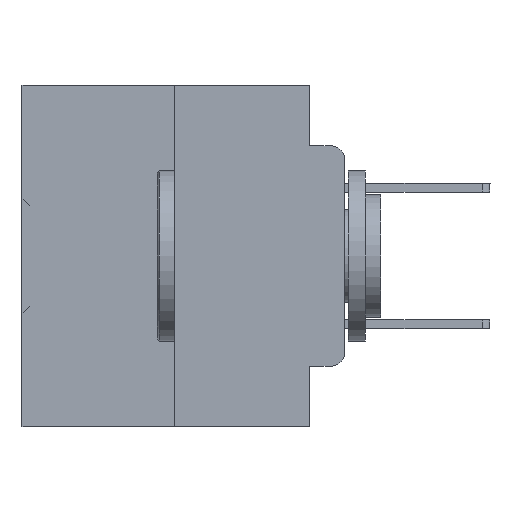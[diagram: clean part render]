
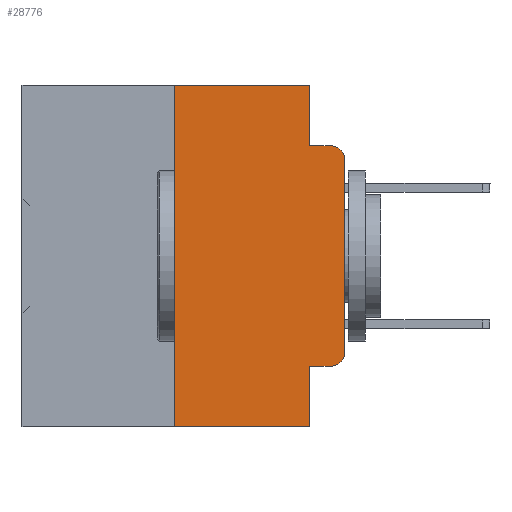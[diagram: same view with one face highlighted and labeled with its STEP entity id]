
A CAD part, left-side view. The second image highlights one B-rep face of the part: STEP entity #28776.
In plain terms, the highlighted planar face has unit normal (-1, 0, 0).
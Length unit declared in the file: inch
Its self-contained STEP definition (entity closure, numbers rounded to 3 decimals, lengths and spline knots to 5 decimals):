
#138 = VERTEX_POINT ( 'NONE', #4780 ) ;
#224 = VERTEX_POINT ( 'NONE', #30484 ) ;
#926 = VERTEX_POINT ( 'NONE', #33487 ) ;
#1005 = FACE_OUTER_BOUND ( 'NONE', #6523, .T. ) ;
#1361 = LINE ( 'NONE', #36546, #33646 ) ;
#1644 = CARTESIAN_POINT ( 'NONE',  ( 0., 0.02, -0.0885 ) ) ;
#2050 = CARTESIAN_POINT ( 'NONE',  ( 0., 0.02, -0.4115 ) ) ;
#2787 = DIRECTION ( 'NONE',  ( 0., 0., -1. ) ) ;
#3544 = EDGE_CURVE ( 'NONE', #7871, #9605, #33905, .T. ) ;
#3563 = ORIENTED_EDGE ( 'NONE', *, *, #5398, .F. ) ;
#4610 = CARTESIAN_POINT ( 'NONE',  ( 0., 0.051, -0.4115 ) ) ;
#4780 = CARTESIAN_POINT ( 'NONE',  ( 0., 0.051, 0. ) ) ;
#4832 = EDGE_CURVE ( 'NONE', #22934, #23309, #10709, .T. ) ;
#5270 = CARTESIAN_POINT ( 'NONE',  ( 0., 0.051, -0.0885 ) ) ;
#5398 = EDGE_CURVE ( 'NONE', #7871, #926, #38630, .T. ) ;
#5554 = CARTESIAN_POINT ( 'NONE',  ( 0., 0.02, -0.1085 ) ) ;
#5625 = LINE ( 'NONE', #5270, #18079 ) ;
#5853 = VECTOR ( 'NONE', #7792, 39.37008 ) ;
#6523 = EDGE_LOOP ( 'NONE', ( #37694, #24678, #22827, #24062, #15178, #3563, #34292, #28513, #22825, #31174 ) ) ;
#6553 = VECTOR ( 'NONE', #20130, 39.37008 ) ;
#6587 = EDGE_CURVE ( 'NONE', #23309, #18038, #19719, .T. ) ;
#7758 = LINE ( 'NONE', #39759, #5853 ) ;
#7762 = EDGE_CURVE ( 'NONE', #21793, #22934, #33129, .T. ) ;
#7792 = DIRECTION ( 'NONE',  ( 0., 0., -1. ) ) ;
#7871 = VERTEX_POINT ( 'NONE', #16027 ) ;
#9605 = VERTEX_POINT ( 'NONE', #36719 ) ;
#9939 = DIRECTION ( 'NONE',  ( 0., -1., 0. ) ) ;
#10709 = LINE ( 'NONE', #34266, #25124 ) ;
#11032 = CARTESIAN_POINT ( 'NONE',  ( 0., 0.473, 0. ) ) ;
#11164 = VECTOR ( 'NONE', #32189, 39.37008 ) ;
#11918 = DIRECTION ( 'NONE',  ( 0., 0., 1. ) ) ;
#14971 = DIRECTION ( 'NONE',  ( 0., 0., -1. ) ) ;
#15178 = ORIENTED_EDGE ( 'NONE', *, *, #18721, .F. ) ;
#15351 = EDGE_CURVE ( 'NONE', #138, #25453, #7758, .T. ) ;
#15486 = DIRECTION ( 'NONE',  ( -1., 0., 0. ) ) ;
#15537 = VECTOR ( 'NONE', #9939, 39.37008 ) ;
#16027 = CARTESIAN_POINT ( 'NONE',  ( 0., 0.25, -0.5 ) ) ;
#16754 = CARTESIAN_POINT ( 'NONE',  ( 0., 0.473, 0. ) ) ;
#17069 = DIRECTION ( 'NONE',  ( 1., 0., 0. ) ) ;
#17585 = DIRECTION ( 'NONE',  ( 0., -1., 0. ) ) ;
#18038 = VERTEX_POINT ( 'NONE', #1644 ) ;
#18079 = VECTOR ( 'NONE', #17585, 39.37008 ) ;
#18721 = EDGE_CURVE ( 'NONE', #926, #138, #27687, .T. ) ;
#18934 = AXIS2_PLACEMENT_3D ( 'NONE', #5554, #33798, #39496 ) ;
#19719 = CIRCLE ( 'NONE', #18934, 0.02 ) ;
#20130 = DIRECTION ( 'NONE',  ( 0., -1., 0. ) ) ;
#21793 = VERTEX_POINT ( 'NONE', #2050 ) ;
#22215 = VECTOR ( 'NONE', #11918, 39.37008 ) ;
#22756 = DIRECTION ( 'NONE',  ( 0., 0., 1. ) ) ;
#22825 = ORIENTED_EDGE ( 'NONE', *, *, #26971, .T. ) ;
#22827 = ORIENTED_EDGE ( 'NONE', *, *, #25513, .F. ) ;
#22934 = VERTEX_POINT ( 'NONE', #28777 ) ;
#23251 = DIRECTION ( 'NONE',  ( 0., 0., -1. ) ) ;
#23309 = VERTEX_POINT ( 'NONE', #24416 ) ;
#24062 = ORIENTED_EDGE ( 'NONE', *, *, #15351, .F. ) ;
#24396 = EDGE_CURVE ( 'NONE', #224, #9605, #1361, .T. ) ;
#24416 = CARTESIAN_POINT ( 'NONE',  ( 0., 0., -0.1085 ) ) ;
#24678 = ORIENTED_EDGE ( 'NONE', *, *, #6587, .T. ) ;
#25124 = VECTOR ( 'NONE', #22756, 39.37008 ) ;
#25453 = VERTEX_POINT ( 'NONE', #31910 ) ;
#25513 = EDGE_CURVE ( 'NONE', #25453, #18038, #5625, .T. ) ;
#26531 = LINE ( 'NONE', #4610, #11164 ) ;
#26590 = PLANE ( 'NONE',  #27819 ) ;
#26971 = EDGE_CURVE ( 'NONE', #224, #21793, #26531, .T. ) ;
#27687 = LINE ( 'NONE', #16754, #6553 ) ;
#27819 = AXIS2_PLACEMENT_3D ( 'NONE', #11032, #17069, #23251 ) ;
#28513 = ORIENTED_EDGE ( 'NONE', *, *, #24396, .F. ) ;
#28776 = ADVANCED_FACE ( 'NONE', ( #1005 ), #26590, .F. ) ;
#28777 = CARTESIAN_POINT ( 'NONE',  ( 0., 0., -0.3915 ) ) ;
#30484 = CARTESIAN_POINT ( 'NONE',  ( 0., 0.051, -0.4115 ) ) ;
#31174 = ORIENTED_EDGE ( 'NONE', *, *, #7762, .T. ) ;
#31494 = CARTESIAN_POINT ( 'NONE',  ( 0., 0.473, -0.5 ) ) ;
#31910 = CARTESIAN_POINT ( 'NONE',  ( 0., 0.051, -0.0885 ) ) ;
#32189 = DIRECTION ( 'NONE',  ( 0., -1., 0. ) ) ;
#33129 = CIRCLE ( 'NONE', #39150, 0.02 ) ;
#33487 = CARTESIAN_POINT ( 'NONE',  ( 0., 0.25, 0. ) ) ;
#33646 = VECTOR ( 'NONE', #14971, 39.37008 ) ;
#33798 = DIRECTION ( 'NONE',  ( -1., 0., 0. ) ) ;
#33905 = LINE ( 'NONE', #31494, #15537 ) ;
#34266 = CARTESIAN_POINT ( 'NONE',  ( 0., 0., 0. ) ) ;
#34292 = ORIENTED_EDGE ( 'NONE', *, *, #3544, .T. ) ;
#36546 = CARTESIAN_POINT ( 'NONE',  ( 0., 0.051, 0. ) ) ;
#36665 = CARTESIAN_POINT ( 'NONE',  ( 0., 0.02, -0.3915 ) ) ;
#36719 = CARTESIAN_POINT ( 'NONE',  ( 0., 0.051, -0.5 ) ) ;
#37694 = ORIENTED_EDGE ( 'NONE', *, *, #4832, .T. ) ;
#38630 = LINE ( 'NONE', #39723, #22215 ) ;
#39150 = AXIS2_PLACEMENT_3D ( 'NONE', #36665, #15486, #2787 ) ;
#39496 = DIRECTION ( 'NONE',  ( 0., 0., -1. ) ) ;
#39723 = CARTESIAN_POINT ( 'NONE',  ( 0., 0.25, 0. ) ) ;
#39759 = CARTESIAN_POINT ( 'NONE',  ( 0., 0.051, 0. ) ) ;
